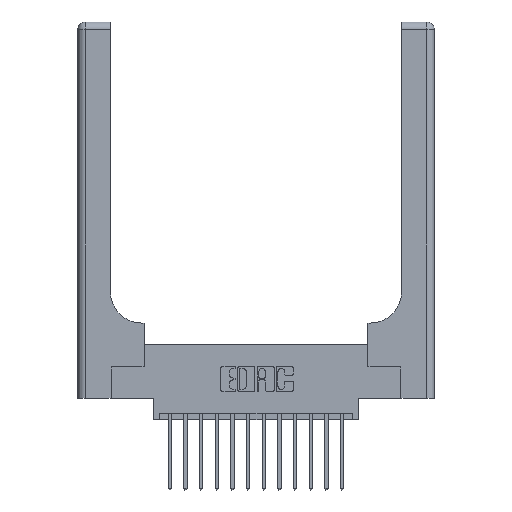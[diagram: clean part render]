
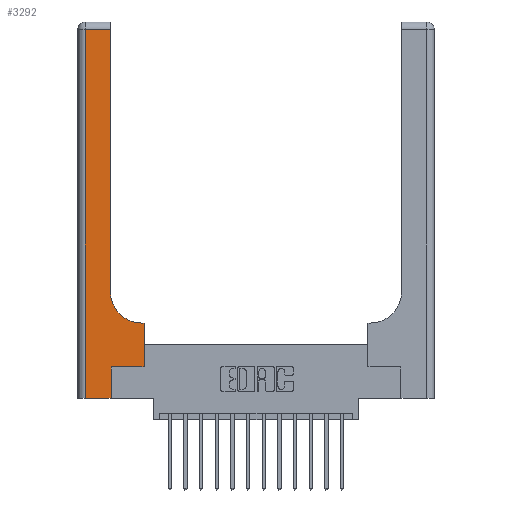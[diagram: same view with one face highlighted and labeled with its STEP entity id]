
A CAD part, top view. The second image highlights one B-rep face of the part: STEP entity #3292.
In plain terms, the highlighted planar face has unit normal (0, 0, 1).
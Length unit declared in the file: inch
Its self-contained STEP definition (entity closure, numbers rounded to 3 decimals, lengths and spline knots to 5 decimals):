
#179 = CARTESIAN_POINT ( 'NONE',  ( 0.265, 0., 0.37 ) ) ;
#194 = AXIS2_PLACEMENT_3D ( 'NONE', #12363, #7113, #13802 ) ;
#203 = DIRECTION ( 'NONE',  ( -1., 0., 0. ) ) ;
#331 = EDGE_CURVE ( 'NONE', #11240, #7622, #8466, .T. ) ;
#433 = DIRECTION ( 'NONE',  ( 0., 1., 0. ) ) ;
#695 = DIRECTION ( 'NONE',  ( 1., 0., 0. ) ) ;
#858 = LINE ( 'NONE', #10571, #14696 ) ;
#1374 = CARTESIAN_POINT ( 'NONE',  ( 0., 0., 0.37 ) ) ;
#1684 = ORIENTED_EDGE ( 'NONE', *, *, #15470, .T. ) ;
#1822 = VERTEX_POINT ( 'NONE', #12509 ) ;
#2018 = VERTEX_POINT ( 'NONE', #10053 ) ;
#2128 = ORIENTED_EDGE ( 'NONE', *, *, #8045, .T. ) ;
#2552 = CARTESIAN_POINT ( 'NONE',  ( 0.265, 0.25, 0.37 ) ) ;
#2602 = ORIENTED_EDGE ( 'NONE', *, *, #5337, .T. ) ;
#2733 = CIRCLE ( 'NONE', #15543, 0.25 ) ;
#2783 = CARTESIAN_POINT ( 'NONE',  ( 0.06, 3., 0.37 ) ) ;
#2890 = ORIENTED_EDGE ( 'NONE', *, *, #11914, .T. ) ;
#3292 = ADVANCED_FACE ( 'NONE', ( #15978 ), #11120, .F. ) ;
#3329 = LINE ( 'NONE', #4590, #4433 ) ;
#3515 = EDGE_CURVE ( 'NONE', #5655, #11240, #858, .T. ) ;
#4353 = CARTESIAN_POINT ( 'NONE',  ( 0.26, 2.94, 0.37 ) ) ;
#4433 = VECTOR ( 'NONE', #10014, 39.37008 ) ;
#4590 = CARTESIAN_POINT ( 'NONE',  ( 0.26, 0.6, 0.37 ) ) ;
#4655 = EDGE_LOOP ( 'NONE', ( #1684, #2890, #9024, #2128, #11655, #12789, #12761, #2602, #10996 ) ) ;
#4715 = EDGE_CURVE ( 'NONE', #17378, #12933, #2733, .T. ) ;
#4773 = VECTOR ( 'NONE', #203, 39.37008 ) ;
#5337 = EDGE_CURVE ( 'NONE', #2018, #17378, #3329, .T. ) ;
#5655 = VERTEX_POINT ( 'NONE', #179 ) ;
#5887 = CARTESIAN_POINT ( 'NONE',  ( 0.265, 0.25, 0.37 ) ) ;
#5912 = LINE ( 'NONE', #16449, #4773 ) ;
#6458 = VERTEX_POINT ( 'NONE', #12272 ) ;
#6846 = EDGE_CURVE ( 'NONE', #1822, #6458, #6964, .T. ) ;
#6964 = LINE ( 'NONE', #2783, #16632 ) ;
#7113 = DIRECTION ( 'NONE',  ( 0., 0., -1. ) ) ;
#7340 = DIRECTION ( 'NONE',  ( 0., 1., 0. ) ) ;
#7465 = VECTOR ( 'NONE', #16693, 39.37008 ) ;
#7622 = VERTEX_POINT ( 'NONE', #8007 ) ;
#7989 = DIRECTION ( 'NONE',  ( 0., 1., 0. ) ) ;
#8007 = CARTESIAN_POINT ( 'NONE',  ( 0.528, 0.25, 0.37 ) ) ;
#8045 = EDGE_CURVE ( 'NONE', #6458, #5655, #13868, .T. ) ;
#8326 = DIRECTION ( 'NONE',  ( 1., 0., 0. ) ) ;
#8466 = LINE ( 'NONE', #5887, #7465 ) ;
#8933 = LINE ( 'NONE', #12687, #9295 ) ;
#9024 = ORIENTED_EDGE ( 'NONE', *, *, #6846, .T. ) ;
#9295 = VECTOR ( 'NONE', #7340, 39.37008 ) ;
#9794 = CARTESIAN_POINT ( 'NONE',  ( 0.528, 0.25, 0.37 ) ) ;
#9911 = DIRECTION ( 'NONE',  ( 0., -1., 0. ) ) ;
#10014 = DIRECTION ( 'NONE',  ( -1., 0., 0. ) ) ;
#10053 = CARTESIAN_POINT ( 'NONE',  ( 0.528, 0.6, 0.37 ) ) ;
#10571 = CARTESIAN_POINT ( 'NONE',  ( 0.265, 0., 0.37 ) ) ;
#10952 = VERTEX_POINT ( 'NONE', #4353 ) ;
#10996 = ORIENTED_EDGE ( 'NONE', *, *, #4715, .T. ) ;
#11015 = VECTOR ( 'NONE', #433, 39.37008 ) ;
#11120 = PLANE ( 'NONE',  #194 ) ;
#11240 = VERTEX_POINT ( 'NONE', #2552 ) ;
#11655 = ORIENTED_EDGE ( 'NONE', *, *, #3515, .T. ) ;
#11914 = EDGE_CURVE ( 'NONE', #10952, #1822, #5912, .T. ) ;
#12272 = CARTESIAN_POINT ( 'NONE',  ( 0.06, 0., 0.37 ) ) ;
#12363 = CARTESIAN_POINT ( 'NONE',  ( 0., 3., 0.37 ) ) ;
#12509 = CARTESIAN_POINT ( 'NONE',  ( 0.06, 2.94, 0.37 ) ) ;
#12645 = LINE ( 'NONE', #9794, #11015 ) ;
#12687 = CARTESIAN_POINT ( 'NONE',  ( 0.26, 3., 0.37 ) ) ;
#12761 = ORIENTED_EDGE ( 'NONE', *, *, #16303, .T. ) ;
#12789 = ORIENTED_EDGE ( 'NONE', *, *, #331, .T. ) ;
#12933 = VERTEX_POINT ( 'NONE', #14117 ) ;
#13101 = CARTESIAN_POINT ( 'NONE',  ( 0.51, 0.85, 0.37 ) ) ;
#13802 = DIRECTION ( 'NONE',  ( -1., 0., 0. ) ) ;
#13868 = LINE ( 'NONE', #1374, #15098 ) ;
#14117 = CARTESIAN_POINT ( 'NONE',  ( 0.26, 0.85, 0.37 ) ) ;
#14269 = DIRECTION ( 'NONE',  ( 0., 0., -1. ) ) ;
#14696 = VECTOR ( 'NONE', #7989, 39.37008 ) ;
#15098 = VECTOR ( 'NONE', #8326, 39.37008 ) ;
#15470 = EDGE_CURVE ( 'NONE', #12933, #10952, #8933, .T. ) ;
#15543 = AXIS2_PLACEMENT_3D ( 'NONE', #13101, #14269, #695 ) ;
#15978 = FACE_OUTER_BOUND ( 'NONE', #4655, .T. ) ;
#16303 = EDGE_CURVE ( 'NONE', #7622, #2018, #12645, .T. ) ;
#16449 = CARTESIAN_POINT ( 'NONE',  ( 0., 2.94, 0.37 ) ) ;
#16632 = VECTOR ( 'NONE', #9911, 39.37008 ) ;
#16693 = DIRECTION ( 'NONE',  ( 1., 0., 0. ) ) ;
#16777 = CARTESIAN_POINT ( 'NONE',  ( 0.51, 0.6, 0.37 ) ) ;
#17378 = VERTEX_POINT ( 'NONE', #16777 ) ;
